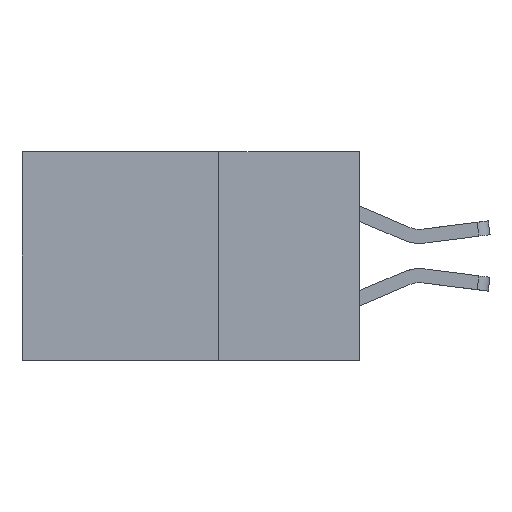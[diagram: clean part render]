
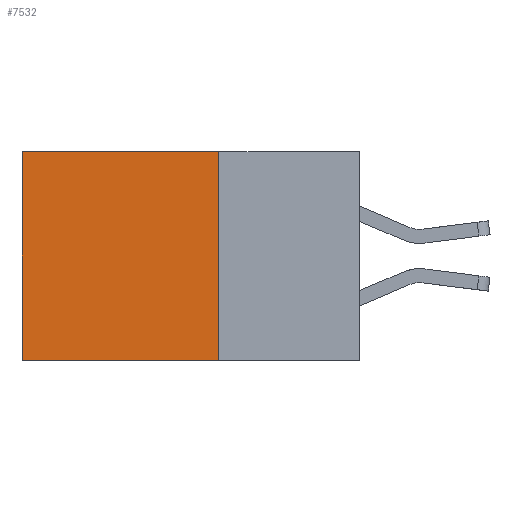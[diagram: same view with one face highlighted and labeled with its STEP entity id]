
A CAD part, left-side view. The second image highlights one B-rep face of the part: STEP entity #7532.
In plain terms, the highlighted planar face has unit normal (-1, 0, 0).
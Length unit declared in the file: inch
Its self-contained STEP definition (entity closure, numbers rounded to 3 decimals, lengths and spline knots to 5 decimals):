
#585 = VERTEX_POINT ( 'NONE', #2147 ) ;
#732 = PLANE ( 'NONE',  #6039 ) ;
#922 = VECTOR ( 'NONE', #9593, 39.37008 ) ;
#981 = CARTESIAN_POINT ( 'NONE',  ( 0.2875, 0.25, 0. ) ) ;
#1383 = EDGE_CURVE ( 'NONE', #4018, #585, #4089, .T. ) ;
#1916 = CARTESIAN_POINT ( 'NONE',  ( 0.2875, 0.25, 0. ) ) ;
#2118 = ORIENTED_EDGE ( 'NONE', *, *, #3502, .F. ) ;
#2147 = CARTESIAN_POINT ( 'NONE',  ( 0.2875, 0.6, -0.37 ) ) ;
#2848 = EDGE_LOOP ( 'NONE', ( #9104, #11785, #2118, #7214 ) ) ;
#3001 = DIRECTION ( 'NONE',  ( 1., 0., 0. ) ) ;
#3153 = VECTOR ( 'NONE', #3717, 39.37008 ) ;
#3502 = EDGE_CURVE ( 'NONE', #6635, #9403, #10878, .T. ) ;
#3506 = DIRECTION ( 'NONE',  ( 0., 0., -1. ) ) ;
#3717 = DIRECTION ( 'NONE',  ( 0., 1., 0. ) ) ;
#3791 = VECTOR ( 'NONE', #3506, 39.37008 ) ;
#3817 = CARTESIAN_POINT ( 'NONE',  ( 0.2875, 0.25, -0.37 ) ) ;
#4018 = VERTEX_POINT ( 'NONE', #6903 ) ;
#4089 = LINE ( 'NONE', #4225, #3791 ) ;
#4225 = CARTESIAN_POINT ( 'NONE',  ( 0.2875, 0.6, 0. ) ) ;
#4303 = EDGE_CURVE ( 'NONE', #9403, #585, #10294, .T. ) ;
#5035 = CARTESIAN_POINT ( 'NONE',  ( 0.2875, 0.25, 0. ) ) ;
#5750 = LINE ( 'NONE', #981, #7855 ) ;
#6039 = AXIS2_PLACEMENT_3D ( 'NONE', #1916, #3001, #9551 ) ;
#6635 = VERTEX_POINT ( 'NONE', #10275 ) ;
#6903 = CARTESIAN_POINT ( 'NONE',  ( 0.2875, 0.6, 0. ) ) ;
#6937 = DIRECTION ( 'NONE',  ( 0., 1., 0. ) ) ;
#7214 = ORIENTED_EDGE ( 'NONE', *, *, #10641, .T. ) ;
#7532 = ADVANCED_FACE ( 'NONE', ( #7917 ), #732, .F. ) ;
#7855 = VECTOR ( 'NONE', #6937, 39.37008 ) ;
#7917 = FACE_OUTER_BOUND ( 'NONE', #2848, .T. ) ;
#9104 = ORIENTED_EDGE ( 'NONE', *, *, #1383, .T. ) ;
#9403 = VERTEX_POINT ( 'NONE', #3817 ) ;
#9551 = DIRECTION ( 'NONE',  ( 0., 0., -1. ) ) ;
#9593 = DIRECTION ( 'NONE',  ( 0., 0., -1. ) ) ;
#10160 = CARTESIAN_POINT ( 'NONE',  ( 0.2875, 0.25, -0.37 ) ) ;
#10275 = CARTESIAN_POINT ( 'NONE',  ( 0.2875, 0.25, 0. ) ) ;
#10294 = LINE ( 'NONE', #10160, #3153 ) ;
#10641 = EDGE_CURVE ( 'NONE', #6635, #4018, #5750, .T. ) ;
#10878 = LINE ( 'NONE', #5035, #922 ) ;
#11785 = ORIENTED_EDGE ( 'NONE', *, *, #4303, .F. ) ;
